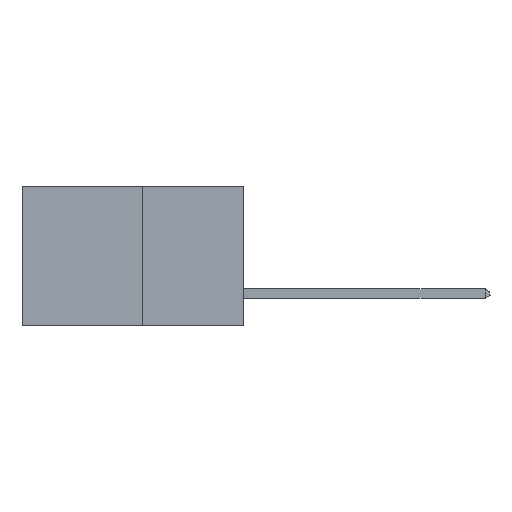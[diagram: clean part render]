
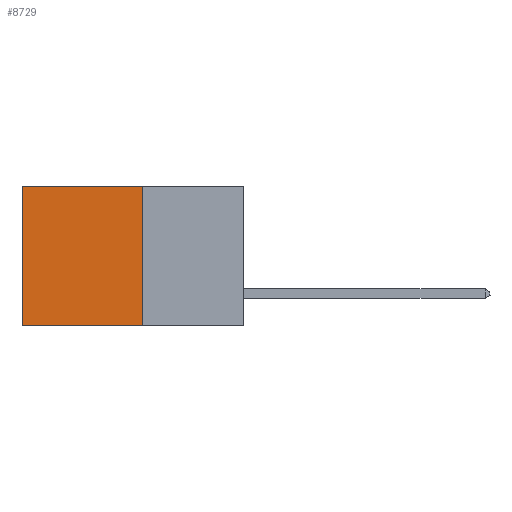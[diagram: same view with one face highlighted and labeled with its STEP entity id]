
A CAD part, left-side view. The second image highlights one B-rep face of the part: STEP entity #8729.
In plain terms, the highlighted planar face has unit normal (-1, 0, 0).
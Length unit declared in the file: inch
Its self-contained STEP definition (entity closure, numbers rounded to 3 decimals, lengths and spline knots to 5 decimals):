
#839 = VECTOR ( 'NONE', #20057, 39.37008 ) ;
#2685 = VERTEX_POINT ( 'NONE', #22997 ) ;
#3050 = VECTOR ( 'NONE', #14026, 39.37008 ) ;
#5652 = CARTESIAN_POINT ( 'NONE',  ( 0.277, 0.59, -0.37 ) ) ;
#5688 = DIRECTION ( 'NONE',  ( 0., 1., 0. ) ) ;
#6064 = PLANE ( 'NONE',  #12298 ) ;
#6100 = VERTEX_POINT ( 'NONE', #22384 ) ;
#6624 = LINE ( 'NONE', #17979, #839 ) ;
#7138 = CARTESIAN_POINT ( 'NONE',  ( 0.277, 0.27, -0.37 ) ) ;
#8090 = LINE ( 'NONE', #5652, #3050 ) ;
#8729 = ADVANCED_FACE ( 'NONE', ( #14217 ), #6064, .F. ) ;
#9674 = EDGE_CURVE ( 'NONE', #15861, #6100, #25357, .T. ) ;
#10493 = VERTEX_POINT ( 'NONE', #26732 ) ;
#12298 = AXIS2_PLACEMENT_3D ( 'NONE', #23052, #25119, #12405 ) ;
#12405 = DIRECTION ( 'NONE',  ( 0., 0., -1. ) ) ;
#14026 = DIRECTION ( 'NONE',  ( 0., 0., -1. ) ) ;
#14079 = VECTOR ( 'NONE', #24209, 39.37008 ) ;
#14217 = FACE_OUTER_BOUND ( 'NONE', #26598, .T. ) ;
#15861 = VERTEX_POINT ( 'NONE', #16662 ) ;
#15966 = ORIENTED_EDGE ( 'NONE', *, *, #25857, .T. ) ;
#16320 = LINE ( 'NONE', #20547, #22008 ) ;
#16662 = CARTESIAN_POINT ( 'NONE',  ( 0.277, 0.27, 0. ) ) ;
#17979 = CARTESIAN_POINT ( 'NONE',  ( 0.277, 0.27, 0. ) ) ;
#20057 = DIRECTION ( 'NONE',  ( 0., 1., 0. ) ) ;
#20194 = ORIENTED_EDGE ( 'NONE', *, *, #20831, .F. ) ;
#20547 = CARTESIAN_POINT ( 'NONE',  ( 0.277, 0.27, -0.37 ) ) ;
#20831 = EDGE_CURVE ( 'NONE', #6100, #2685, #16320, .T. ) ;
#22008 = VECTOR ( 'NONE', #5688, 39.37008 ) ;
#22384 = CARTESIAN_POINT ( 'NONE',  ( 0.277, 0.27, -0.37 ) ) ;
#22451 = ORIENTED_EDGE ( 'NONE', *, *, #9674, .F. ) ;
#22997 = CARTESIAN_POINT ( 'NONE',  ( 0.277, 0.59, -0.37 ) ) ;
#23052 = CARTESIAN_POINT ( 'NONE',  ( 0.277, 0.27, -0.37 ) ) ;
#24209 = DIRECTION ( 'NONE',  ( 0., 0., -1. ) ) ;
#24484 = ORIENTED_EDGE ( 'NONE', *, *, #27487, .T. ) ;
#25119 = DIRECTION ( 'NONE',  ( 1., 0., 0. ) ) ;
#25357 = LINE ( 'NONE', #7138, #14079 ) ;
#25857 = EDGE_CURVE ( 'NONE', #10493, #2685, #8090, .T. ) ;
#26598 = EDGE_LOOP ( 'NONE', ( #15966, #20194, #22451, #24484 ) ) ;
#26732 = CARTESIAN_POINT ( 'NONE',  ( 0.277, 0.59, 0. ) ) ;
#27487 = EDGE_CURVE ( 'NONE', #15861, #10493, #6624, .T. ) ;
